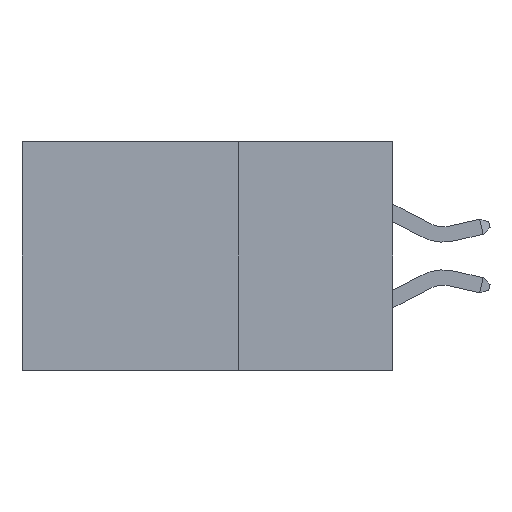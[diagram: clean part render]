
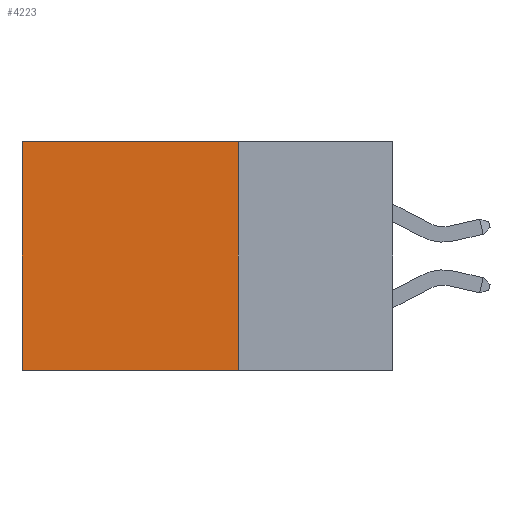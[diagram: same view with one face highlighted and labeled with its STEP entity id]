
A CAD part, left-side view. The second image highlights one B-rep face of the part: STEP entity #4223.
In plain terms, the highlighted planar face has unit normal (-1, 0, 0).
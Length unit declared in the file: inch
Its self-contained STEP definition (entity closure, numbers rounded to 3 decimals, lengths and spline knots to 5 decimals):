
#1099 = DIRECTION ( 'NONE',  ( 0., 0., -1. ) ) ;
#1251 = CARTESIAN_POINT ( 'NONE',  ( 0.2875, 0.25, -0.37 ) ) ;
#3047 = LINE ( 'NONE', #1251, #7032 ) ;
#3596 = DIRECTION ( 'NONE',  ( 0., 1., 0. ) ) ;
#3965 = LINE ( 'NONE', #12091, #16409 ) ;
#4223 = ADVANCED_FACE ( 'NONE', ( #12339 ), #19638, .F. ) ;
#4292 = EDGE_CURVE ( 'NONE', #21912, #4642, #3047, .T. ) ;
#4626 = CARTESIAN_POINT ( 'NONE',  ( 0.2875, 0.25, 0. ) ) ;
#4642 = VERTEX_POINT ( 'NONE', #9000 ) ;
#5437 = ORIENTED_EDGE ( 'NONE', *, *, #21624, .T. ) ;
#7032 = VECTOR ( 'NONE', #14885, 39.37008 ) ;
#7944 = CARTESIAN_POINT ( 'NONE',  ( 0.2875, 0.25, 0. ) ) ;
#9000 = CARTESIAN_POINT ( 'NONE',  ( 0.2875, 0.6, -0.37 ) ) ;
#9480 = DIRECTION ( 'NONE',  ( 0., 0., -1. ) ) ;
#10897 = VERTEX_POINT ( 'NONE', #15192 ) ;
#11381 = DIRECTION ( 'NONE',  ( 1., 0., 0. ) ) ;
#12091 = CARTESIAN_POINT ( 'NONE',  ( 0.2875, 0.25, 0. ) ) ;
#12104 = VECTOR ( 'NONE', #9480, 39.37008 ) ;
#12339 = FACE_OUTER_BOUND ( 'NONE', #13824, .T. ) ;
#12631 = LINE ( 'NONE', #21180, #12104 ) ;
#13417 = CARTESIAN_POINT ( 'NONE',  ( 0.2875, 0.6, 0. ) ) ;
#13824 = EDGE_LOOP ( 'NONE', ( #14911, #14430, #19331, #5437 ) ) ;
#14430 = ORIENTED_EDGE ( 'NONE', *, *, #4292, .F. ) ;
#14778 = DIRECTION ( 'NONE',  ( 0., 0., -1. ) ) ;
#14863 = EDGE_CURVE ( 'NONE', #21474, #4642, #12631, .T. ) ;
#14885 = DIRECTION ( 'NONE',  ( 0., 1., 0. ) ) ;
#14898 = LINE ( 'NONE', #4626, #18810 ) ;
#14911 = ORIENTED_EDGE ( 'NONE', *, *, #14863, .T. ) ;
#15192 = CARTESIAN_POINT ( 'NONE',  ( 0.2875, 0.25, 0. ) ) ;
#15895 = CARTESIAN_POINT ( 'NONE',  ( 0.2875, 0.25, -0.37 ) ) ;
#16409 = VECTOR ( 'NONE', #3596, 39.37008 ) ;
#17365 = EDGE_CURVE ( 'NONE', #10897, #21912, #14898, .T. ) ;
#18810 = VECTOR ( 'NONE', #14778, 39.37008 ) ;
#19331 = ORIENTED_EDGE ( 'NONE', *, *, #17365, .F. ) ;
#19638 = PLANE ( 'NONE',  #19939 ) ;
#19939 = AXIS2_PLACEMENT_3D ( 'NONE', #7944, #11381, #1099 ) ;
#21180 = CARTESIAN_POINT ( 'NONE',  ( 0.2875, 0.6, 0. ) ) ;
#21474 = VERTEX_POINT ( 'NONE', #13417 ) ;
#21624 = EDGE_CURVE ( 'NONE', #10897, #21474, #3965, .T. ) ;
#21912 = VERTEX_POINT ( 'NONE', #15895 ) ;
